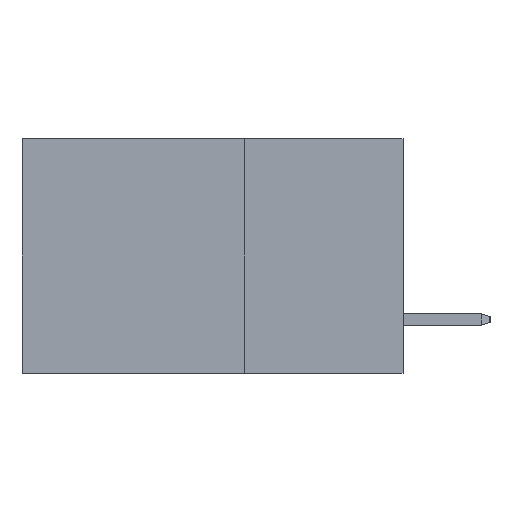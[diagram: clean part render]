
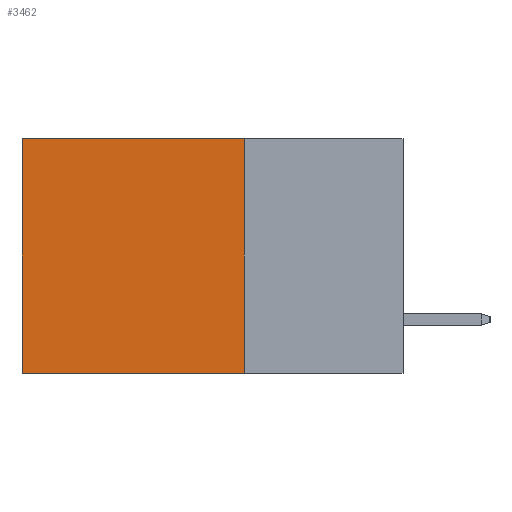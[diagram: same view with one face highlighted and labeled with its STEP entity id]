
A CAD part, left-side view. The second image highlights one B-rep face of the part: STEP entity #3462.
In plain terms, the highlighted planar face has unit normal (-1, 0, 0).
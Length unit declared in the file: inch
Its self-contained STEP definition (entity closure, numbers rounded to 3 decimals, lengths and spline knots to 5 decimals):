
#36 = DIRECTION ( 'NONE',  ( 0., 1., 0. ) ) ;
#84 = CARTESIAN_POINT ( 'NONE',  ( 0.2875, 0.25, 0. ) ) ;
#1203 = DIRECTION ( 'NONE',  ( 0., 1., 0. ) ) ;
#2872 = ORIENTED_EDGE ( 'NONE', *, *, #14485, .T. ) ;
#3240 = VERTEX_POINT ( 'NONE', #8736 ) ;
#3462 = ADVANCED_FACE ( 'NONE', ( #5578 ), #13628, .F. ) ;
#4150 = DIRECTION ( 'NONE',  ( 1., 0., 0. ) ) ;
#5087 = LINE ( 'NONE', #9845, #9516 ) ;
#5295 = ORIENTED_EDGE ( 'NONE', *, *, #8658, .F. ) ;
#5578 = FACE_OUTER_BOUND ( 'NONE', #14819, .T. ) ;
#6007 = CARTESIAN_POINT ( 'NONE',  ( 0.2875, 0.6, -0.37 ) ) ;
#6047 = DIRECTION ( 'NONE',  ( 0., 0., -1. ) ) ;
#6456 = CARTESIAN_POINT ( 'NONE',  ( 0.2875, 0.25, 0. ) ) ;
#6471 = VECTOR ( 'NONE', #15478, 39.37008 ) ;
#6540 = DIRECTION ( 'NONE',  ( 0., 0., -1. ) ) ;
#6916 = VERTEX_POINT ( 'NONE', #8425 ) ;
#7248 = LINE ( 'NONE', #10874, #7649 ) ;
#7351 = VERTEX_POINT ( 'NONE', #12192 ) ;
#7649 = VECTOR ( 'NONE', #36, 39.37008 ) ;
#8425 = CARTESIAN_POINT ( 'NONE',  ( 0.2875, 0.25, -0.37 ) ) ;
#8658 = EDGE_CURVE ( 'NONE', #6916, #14948, #7248, .T. ) ;
#8736 = CARTESIAN_POINT ( 'NONE',  ( 0.2875, 0.6, 0. ) ) ;
#9516 = VECTOR ( 'NONE', #6047, 39.37008 ) ;
#9845 = CARTESIAN_POINT ( 'NONE',  ( 0.2875, 0.6, 0. ) ) ;
#10874 = CARTESIAN_POINT ( 'NONE',  ( 0.2875, 0.25, -0.37 ) ) ;
#11003 = VECTOR ( 'NONE', #1203, 39.37008 ) ;
#11076 = LINE ( 'NONE', #84, #11003 ) ;
#11513 = AXIS2_PLACEMENT_3D ( 'NONE', #6456, #4150, #6540 ) ;
#12192 = CARTESIAN_POINT ( 'NONE',  ( 0.2875, 0.25, 0. ) ) ;
#12479 = ORIENTED_EDGE ( 'NONE', *, *, #12849, .T. ) ;
#12849 = EDGE_CURVE ( 'NONE', #3240, #14948, #5087, .T. ) ;
#12868 = CARTESIAN_POINT ( 'NONE',  ( 0.2875, 0.25, 0. ) ) ;
#13628 = PLANE ( 'NONE',  #11513 ) ;
#14130 = LINE ( 'NONE', #12868, #6471 ) ;
#14227 = ORIENTED_EDGE ( 'NONE', *, *, #14729, .F. ) ;
#14485 = EDGE_CURVE ( 'NONE', #7351, #3240, #11076, .T. ) ;
#14729 = EDGE_CURVE ( 'NONE', #7351, #6916, #14130, .T. ) ;
#14819 = EDGE_LOOP ( 'NONE', ( #12479, #5295, #14227, #2872 ) ) ;
#14948 = VERTEX_POINT ( 'NONE', #6007 ) ;
#15478 = DIRECTION ( 'NONE',  ( 0., 0., -1. ) ) ;
